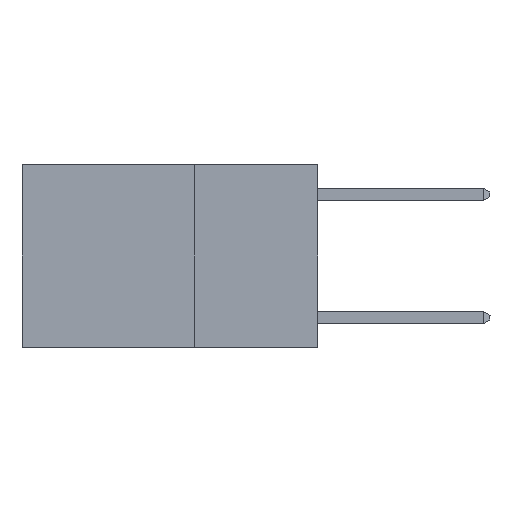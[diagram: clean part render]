
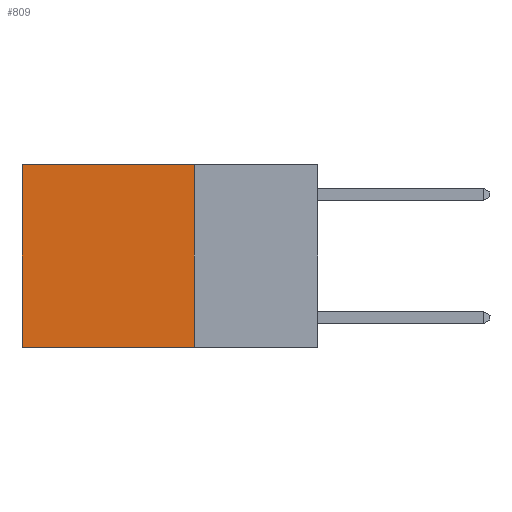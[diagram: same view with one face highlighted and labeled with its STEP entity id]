
A CAD part, left-side view. The second image highlights one B-rep face of the part: STEP entity #809.
In plain terms, the highlighted planar face has unit normal (-1, 0, 0).
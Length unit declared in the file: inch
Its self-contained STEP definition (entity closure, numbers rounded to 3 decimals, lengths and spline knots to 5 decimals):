
#647 = VECTOR ( 'NONE', #8708, 39.37008 ) ;
#809 = ADVANCED_FACE ( 'NONE', ( #11010 ), #11970, .F. ) ;
#1932 = EDGE_LOOP ( 'NONE', ( #7900, #8871, #13752, #11864 ) ) ;
#2554 = EDGE_CURVE ( 'NONE', #13952, #13437, #4180, .T. ) ;
#3107 = CARTESIAN_POINT ( 'NONE',  ( 0.2625, 0.25, 0. ) ) ;
#3912 = EDGE_CURVE ( 'NONE', #10102, #16133, #8055, .T. ) ;
#4180 = LINE ( 'NONE', #16205, #647 ) ;
#4523 = CARTESIAN_POINT ( 'NONE',  ( 0.2625, 0.6, 0. ) ) ;
#4601 = DIRECTION ( 'NONE',  ( 1., 0., 0. ) ) ;
#5383 = LINE ( 'NONE', #13926, #9335 ) ;
#5945 = DIRECTION ( 'NONE',  ( 0., 1., 0. ) ) ;
#7900 = ORIENTED_EDGE ( 'NONE', *, *, #3912, .T. ) ;
#8055 = LINE ( 'NONE', #4523, #8521 ) ;
#8151 = EDGE_CURVE ( 'NONE', #13952, #10102, #16494, .T. ) ;
#8357 = CARTESIAN_POINT ( 'NONE',  ( 0.2625, 0.25, -0.37 ) ) ;
#8521 = VECTOR ( 'NONE', #13410, 39.37008 ) ;
#8708 = DIRECTION ( 'NONE',  ( 0., 0., -1. ) ) ;
#8871 = ORIENTED_EDGE ( 'NONE', *, *, #19116, .F. ) ;
#9335 = VECTOR ( 'NONE', #15458, 39.37008 ) ;
#10102 = VERTEX_POINT ( 'NONE', #16086 ) ;
#10333 = CARTESIAN_POINT ( 'NONE',  ( 0.2625, 0.25, 0. ) ) ;
#10944 = AXIS2_PLACEMENT_3D ( 'NONE', #3107, #4601, #15017 ) ;
#11010 = FACE_OUTER_BOUND ( 'NONE', #1932, .T. ) ;
#11864 = ORIENTED_EDGE ( 'NONE', *, *, #8151, .T. ) ;
#11970 = PLANE ( 'NONE',  #10944 ) ;
#13410 = DIRECTION ( 'NONE',  ( 0., 0., -1. ) ) ;
#13437 = VERTEX_POINT ( 'NONE', #8357 ) ;
#13752 = ORIENTED_EDGE ( 'NONE', *, *, #2554, .F. ) ;
#13926 = CARTESIAN_POINT ( 'NONE',  ( 0.2625, 0.25, -0.37 ) ) ;
#13952 = VERTEX_POINT ( 'NONE', #15558 ) ;
#15017 = DIRECTION ( 'NONE',  ( 0., 0., -1. ) ) ;
#15458 = DIRECTION ( 'NONE',  ( 0., 1., 0. ) ) ;
#15558 = CARTESIAN_POINT ( 'NONE',  ( 0.2625, 0.25, 0. ) ) ;
#16086 = CARTESIAN_POINT ( 'NONE',  ( 0.2625, 0.6, 0. ) ) ;
#16133 = VERTEX_POINT ( 'NONE', #16597 ) ;
#16205 = CARTESIAN_POINT ( 'NONE',  ( 0.2625, 0.25, 0. ) ) ;
#16494 = LINE ( 'NONE', #10333, #16958 ) ;
#16597 = CARTESIAN_POINT ( 'NONE',  ( 0.2625, 0.6, -0.37 ) ) ;
#16958 = VECTOR ( 'NONE', #5945, 39.37008 ) ;
#19116 = EDGE_CURVE ( 'NONE', #13437, #16133, #5383, .T. ) ;
